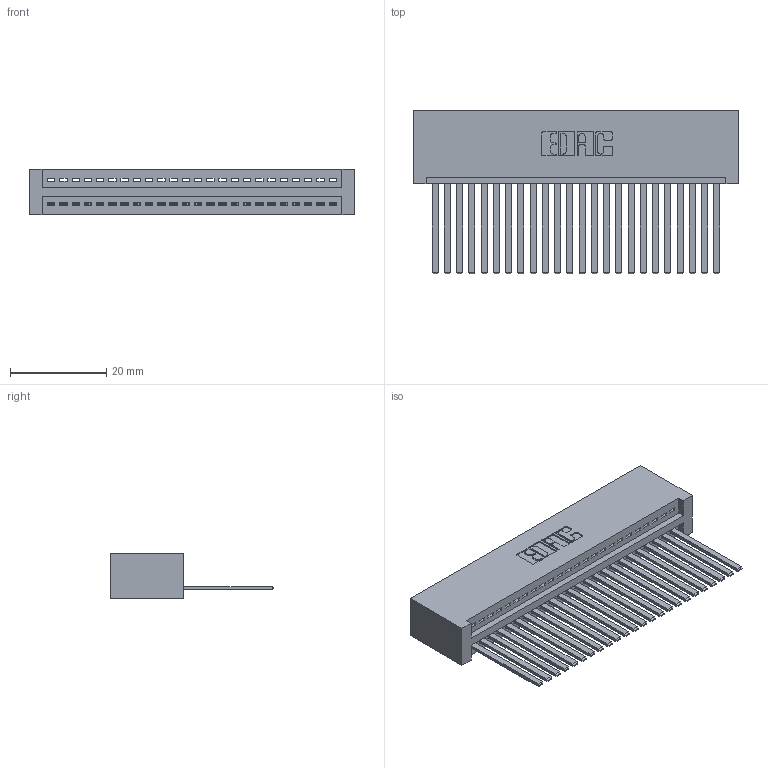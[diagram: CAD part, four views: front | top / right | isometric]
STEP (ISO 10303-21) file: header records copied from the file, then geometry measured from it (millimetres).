
FILE_DESCRIPTION (( 'STEP AP203' ), '1' );
FILE_NAME ('345-024-544-101.STEP', '2019-10-05T05:11:07', ( '' ), ( '' ), 'SwSTEP 2.0', 'SolidWorks 2016', '' );
FILE_SCHEMA (( 'CONFIG_CONTROL_DESIGN' ));
Length unit declared in the file: inch
Products named in the file (3): 345-292-001_345-293-144; 345-024-544-101; 345 Part_No Mounting Lugs
Assembly tree (25 placements, depth 2):
  345-024-544-101
    345 Part_No Mounting Lugs
    345-292-001_345-293-144  x24
Bounding box: 67.56 x 33.96 x 9.4 mm (x, y, z)
Volume: 7132.2 mm3; surface area: 10257.9 mm2
Topology: 25 solids, 25 shells, 1366 faces, 4109 edges, 2706 vertices
Faces by surface type: plane 940, cylinder 426
Entity records: 20025 total; most frequent: CARTESIAN_POINT 3476, ORIENTED_EDGE 3434, DIRECTION 3053, EDGE_CURVE 1717, VECTOR 1501, LINE 1501, VERTEX_POINT 1142, AXIS2_PLACEMENT_3D 776
